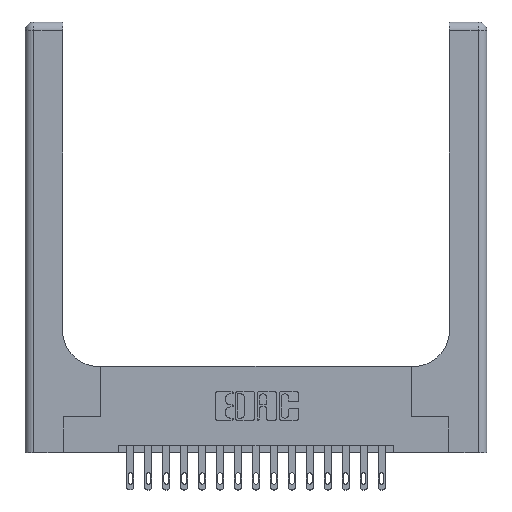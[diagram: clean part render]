
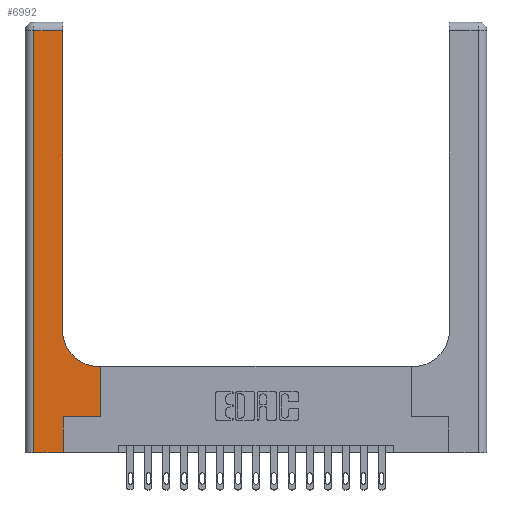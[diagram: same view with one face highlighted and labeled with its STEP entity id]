
A CAD part, top view. The second image highlights one B-rep face of the part: STEP entity #6992.
In plain terms, the highlighted planar face has unit normal (0, 0, 1).
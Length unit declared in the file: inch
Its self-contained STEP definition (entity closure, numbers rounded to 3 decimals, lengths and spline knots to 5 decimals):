
#195 = CARTESIAN_POINT ( 'NONE',  ( 0.265, 0., 0.37 ) ) ;
#539 = VECTOR ( 'NONE', #18352, 39.37008 ) ;
#569 = VERTEX_POINT ( 'NONE', #9226 ) ;
#611 = EDGE_CURVE ( 'NONE', #10555, #13590, #16709, .T. ) ;
#707 = LINE ( 'NONE', #2438, #15369 ) ;
#996 = LINE ( 'NONE', #12736, #13034 ) ;
#1075 = VECTOR ( 'NONE', #14249, 39.37008 ) ;
#1477 = CARTESIAN_POINT ( 'NONE',  ( 0., 3., 0.37 ) ) ;
#1521 = VERTEX_POINT ( 'NONE', #18392 ) ;
#1848 = ORIENTED_EDGE ( 'NONE', *, *, #8200, .T. ) ;
#2088 = CARTESIAN_POINT ( 'NONE',  ( 0.06, 3., 0.37 ) ) ;
#2403 = CARTESIAN_POINT ( 'NONE',  ( 0.06, 2.94, 0.37 ) ) ;
#2438 = CARTESIAN_POINT ( 'NONE',  ( 0., 0., 0.37 ) ) ;
#2915 = DIRECTION ( 'NONE',  ( 0., 0., -1. ) ) ;
#2950 = VECTOR ( 'NONE', #11993, 39.37008 ) ;
#3086 = VERTEX_POINT ( 'NONE', #5100 ) ;
#3549 = DIRECTION ( 'NONE',  ( 0., 1., 0. ) ) ;
#3780 = ORIENTED_EDGE ( 'NONE', *, *, #611, .T. ) ;
#4372 = FACE_OUTER_BOUND ( 'NONE', #7326, .T. ) ;
#4414 = ORIENTED_EDGE ( 'NONE', *, *, #9144, .T. ) ;
#4645 = CARTESIAN_POINT ( 'NONE',  ( 0.265, 0.25, 0.37 ) ) ;
#4867 = VERTEX_POINT ( 'NONE', #10263 ) ;
#5068 = VECTOR ( 'NONE', #17481, 39.37008 ) ;
#5100 = CARTESIAN_POINT ( 'NONE',  ( 0.26, 2.94, 0.37 ) ) ;
#5154 = DIRECTION ( 'NONE',  ( -1., 0., 0. ) ) ;
#5536 = PLANE ( 'NONE',  #6957 ) ;
#5676 = LINE ( 'NONE', #7220, #5068 ) ;
#5689 = ORIENTED_EDGE ( 'NONE', *, *, #17016, .T. ) ;
#6080 = VECTOR ( 'NONE', #3549, 39.37008 ) ;
#6232 = EDGE_CURVE ( 'NONE', #16761, #8755, #15256, .T. ) ;
#6957 = AXIS2_PLACEMENT_3D ( 'NONE', #1477, #2915, #8790 ) ;
#6992 = ADVANCED_FACE ( 'NONE', ( #4372 ), #5536, .F. ) ;
#7220 = CARTESIAN_POINT ( 'NONE',  ( 0.26, 0.6, 0.37 ) ) ;
#7326 = EDGE_LOOP ( 'NONE', ( #14144, #1848, #15894, #17819, #18550, #17940, #3780, #4414, #5689 ) ) ;
#7709 = DIRECTION ( 'NONE',  ( 1., 0., 0. ) ) ;
#8200 = EDGE_CURVE ( 'NONE', #3086, #16761, #996, .T. ) ;
#8755 = VERTEX_POINT ( 'NONE', #12998 ) ;
#8790 = DIRECTION ( 'NONE',  ( -1., 0., 0. ) ) ;
#8977 = EDGE_CURVE ( 'NONE', #1521, #10555, #9050, .T. ) ;
#9050 = LINE ( 'NONE', #4645, #9350 ) ;
#9144 = EDGE_CURVE ( 'NONE', #13590, #569, #5676, .T. ) ;
#9213 = AXIS2_PLACEMENT_3D ( 'NONE', #18149, #13638, #16530 ) ;
#9226 = CARTESIAN_POINT ( 'NONE',  ( 0.51, 0.6, 0.37 ) ) ;
#9350 = VECTOR ( 'NONE', #7709, 39.37008 ) ;
#9414 = CARTESIAN_POINT ( 'NONE',  ( 0.528, 0.25, 0.37 ) ) ;
#9424 = CARTESIAN_POINT ( 'NONE',  ( 0.26, 3., 0.37 ) ) ;
#9847 = EDGE_CURVE ( 'NONE', #13596, #1521, #13958, .T. ) ;
#10263 = CARTESIAN_POINT ( 'NONE',  ( 0.26, 0.85, 0.37 ) ) ;
#10555 = VERTEX_POINT ( 'NONE', #13856 ) ;
#11993 = DIRECTION ( 'NONE',  ( 0., -1., 0. ) ) ;
#12111 = LINE ( 'NONE', #9424, #539 ) ;
#12195 = EDGE_CURVE ( 'NONE', #4867, #3086, #12111, .T. ) ;
#12539 = DIRECTION ( 'NONE',  ( 1., 0., 0. ) ) ;
#12718 = CARTESIAN_POINT ( 'NONE',  ( 0.265, 0., 0.37 ) ) ;
#12736 = CARTESIAN_POINT ( 'NONE',  ( 0., 2.94, 0.37 ) ) ;
#12998 = CARTESIAN_POINT ( 'NONE',  ( 0.06, 0., 0.37 ) ) ;
#13034 = VECTOR ( 'NONE', #5154, 39.37008 ) ;
#13590 = VERTEX_POINT ( 'NONE', #17863 ) ;
#13596 = VERTEX_POINT ( 'NONE', #195 ) ;
#13638 = DIRECTION ( 'NONE',  ( 0., 0., -1. ) ) ;
#13856 = CARTESIAN_POINT ( 'NONE',  ( 0.528, 0.25, 0.37 ) ) ;
#13958 = LINE ( 'NONE', #12718, #1075 ) ;
#14144 = ORIENTED_EDGE ( 'NONE', *, *, #12195, .T. ) ;
#14249 = DIRECTION ( 'NONE',  ( 0., 1., 0. ) ) ;
#15256 = LINE ( 'NONE', #2088, #2950 ) ;
#15369 = VECTOR ( 'NONE', #12539, 39.37008 ) ;
#15894 = ORIENTED_EDGE ( 'NONE', *, *, #6232, .T. ) ;
#16530 = DIRECTION ( 'NONE',  ( 1., 0., 0. ) ) ;
#16709 = LINE ( 'NONE', #9414, #6080 ) ;
#16761 = VERTEX_POINT ( 'NONE', #2403 ) ;
#17016 = EDGE_CURVE ( 'NONE', #569, #4867, #17795, .T. ) ;
#17481 = DIRECTION ( 'NONE',  ( -1., 0., 0. ) ) ;
#17795 = CIRCLE ( 'NONE', #9213, 0.25 ) ;
#17819 = ORIENTED_EDGE ( 'NONE', *, *, #18547, .T. ) ;
#17863 = CARTESIAN_POINT ( 'NONE',  ( 0.528, 0.6, 0.37 ) ) ;
#17940 = ORIENTED_EDGE ( 'NONE', *, *, #8977, .T. ) ;
#18149 = CARTESIAN_POINT ( 'NONE',  ( 0.51, 0.85, 0.37 ) ) ;
#18352 = DIRECTION ( 'NONE',  ( 0., 1., 0. ) ) ;
#18392 = CARTESIAN_POINT ( 'NONE',  ( 0.265, 0.25, 0.37 ) ) ;
#18547 = EDGE_CURVE ( 'NONE', #8755, #13596, #707, .T. ) ;
#18550 = ORIENTED_EDGE ( 'NONE', *, *, #9847, .T. ) ;
